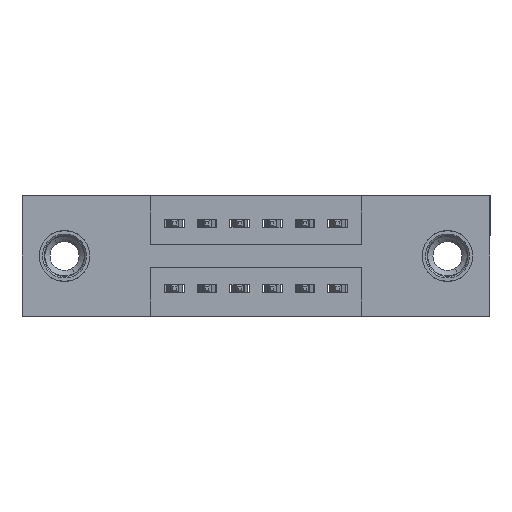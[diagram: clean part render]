
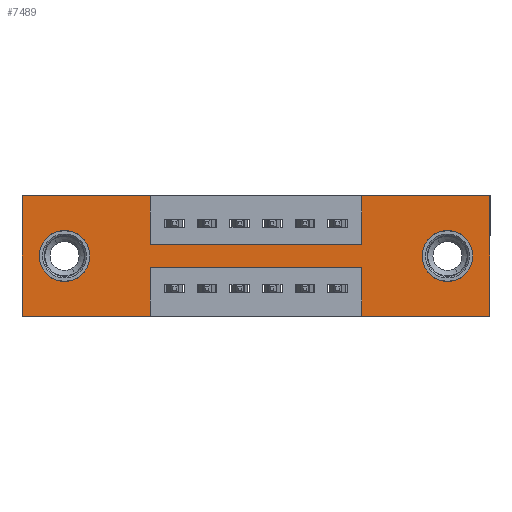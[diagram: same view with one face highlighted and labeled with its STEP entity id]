
A CAD part, front view. The second image highlights one B-rep face of the part: STEP entity #7489.
In plain terms, the highlighted planar face has unit normal (0, -1, 0).
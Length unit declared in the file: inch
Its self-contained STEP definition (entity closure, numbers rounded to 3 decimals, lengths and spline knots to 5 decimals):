
#26 = EDGE_CURVE ( 'NONE', #7139, #14259, #8707, .T. ) ;
#125 = ORIENTED_EDGE ( 'NONE', *, *, #11807, .F. ) ;
#130 = EDGE_CURVE ( 'NONE', #8347, #7900, #1981, .T. ) ;
#423 = VERTEX_POINT ( 'NONE', #5772 ) ;
#432 = LINE ( 'NONE', #14017, #3225 ) ;
#647 = DIRECTION ( 'NONE',  ( 0., 0., 1. ) ) ;
#673 = DIRECTION ( 'NONE',  ( 0., 0., 1. ) ) ;
#773 = VERTEX_POINT ( 'NONE', #10012 ) ;
#780 = DIRECTION ( 'NONE',  ( 1., 0., 0. ) ) ;
#805 = DIRECTION ( 'NONE',  ( 0., 0., -1. ) ) ;
#815 = VECTOR ( 'NONE', #3861, 39.37008 ) ;
#1123 = CARTESIAN_POINT ( 'NONE',  ( 0.3925, 0., -0.37 ) ) ;
#1194 = CARTESIAN_POINT ( 'NONE',  ( 0.3925, 0., 0. ) ) ;
#1325 = EDGE_CURVE ( 'NONE', #8647, #3098, #4925, .T. ) ;
#1399 = ORIENTED_EDGE ( 'NONE', *, *, #7856, .F. ) ;
#1472 = DIRECTION ( 'NONE',  ( -1., 0., 0. ) ) ;
#1557 = LINE ( 'NONE', #3007, #12269 ) ;
#1626 = AXIS2_PLACEMENT_3D ( 'NONE', #12969, #5193, #4157 ) ;
#1705 = ORIENTED_EDGE ( 'NONE', *, *, #10579, .F. ) ;
#1867 = CIRCLE ( 'NONE', #9782, 0.078 ) ;
#1916 = DIRECTION ( 'NONE',  ( 0., 0., -1. ) ) ;
#1981 = CIRCLE ( 'NONE', #10982, 0.078 ) ;
#1982 = VERTEX_POINT ( 'NONE', #1123 ) ;
#2013 = CARTESIAN_POINT ( 'NONE',  ( 1.0425, 0., 0. ) ) ;
#2030 = VECTOR ( 'NONE', #7546, 39.37008 ) ;
#2042 = DIRECTION ( 'NONE',  ( 0., 0., -1. ) ) ;
#2120 = CARTESIAN_POINT ( 'NONE',  ( 1.0425, 0., -0.22 ) ) ;
#2320 = CARTESIAN_POINT ( 'NONE',  ( 0., 0., 0. ) ) ;
#2398 = ORIENTED_EDGE ( 'NONE', *, *, #130, .T. ) ;
#2782 = CARTESIAN_POINT ( 'NONE',  ( 0.3925, 0., -0.22 ) ) ;
#2794 = CARTESIAN_POINT ( 'NONE',  ( 1.0425, 0., 0. ) ) ;
#2824 = EDGE_CURVE ( 'NONE', #14259, #8647, #2837, .T. ) ;
#2837 = LINE ( 'NONE', #7386, #13519 ) ;
#2948 = LINE ( 'NONE', #7271, #6345 ) ;
#3007 = CARTESIAN_POINT ( 'NONE',  ( 1.435, 0., 0. ) ) ;
#3098 = VERTEX_POINT ( 'NONE', #8872 ) ;
#3194 = CARTESIAN_POINT ( 'NONE',  ( 0.13, 0., -0.185 ) ) ;
#3225 = VECTOR ( 'NONE', #11664, 39.37008 ) ;
#3326 = DIRECTION ( 'NONE',  ( 0., 1., 0. ) ) ;
#3330 = ORIENTED_EDGE ( 'NONE', *, *, #9464, .T. ) ;
#3466 = CARTESIAN_POINT ( 'NONE',  ( 1.305, 0., -0.263 ) ) ;
#3505 = CARTESIAN_POINT ( 'NONE',  ( 1.305, 0., -0.185 ) ) ;
#3598 = CARTESIAN_POINT ( 'NONE',  ( 1.0425, 0., -0.37 ) ) ;
#3642 = DIRECTION ( 'NONE',  ( 0., 1., 0. ) ) ;
#3861 = DIRECTION ( 'NONE',  ( -1., 0., 0. ) ) ;
#4094 = FACE_OUTER_BOUND ( 'NONE', #10995, .T. ) ;
#4157 = DIRECTION ( 'NONE',  ( 0., 0., -1. ) ) ;
#4334 = AXIS2_PLACEMENT_3D ( 'NONE', #3505, #3642, #7861 ) ;
#4424 = LINE ( 'NONE', #9378, #815 ) ;
#4527 = VECTOR ( 'NONE', #2042, 39.37008 ) ;
#4878 = VERTEX_POINT ( 'NONE', #7983 ) ;
#4925 = LINE ( 'NONE', #9802, #2030 ) ;
#4985 = ORIENTED_EDGE ( 'NONE', *, *, #6591, .F. ) ;
#5040 = CIRCLE ( 'NONE', #6045, 0.078 ) ;
#5052 = CARTESIAN_POINT ( 'NONE',  ( 0.13, 0., -0.107 ) ) ;
#5193 = DIRECTION ( 'NONE',  ( 0., -1., 0. ) ) ;
#5353 = ORIENTED_EDGE ( 'NONE', *, *, #13831, .F. ) ;
#5372 = ORIENTED_EDGE ( 'NONE', *, *, #7749, .F. ) ;
#5481 = VECTOR ( 'NONE', #9433, 39.37008 ) ;
#5742 = LINE ( 'NONE', #10903, #4527 ) ;
#5757 = EDGE_CURVE ( 'NONE', #7882, #13334, #2948, .T. ) ;
#5772 = CARTESIAN_POINT ( 'NONE',  ( 0.3925, 0., -0.22 ) ) ;
#6045 = AXIS2_PLACEMENT_3D ( 'NONE', #6764, #3326, #6701 ) ;
#6271 = CARTESIAN_POINT ( 'NONE',  ( 1.305, 0., -0.107 ) ) ;
#6345 = VECTOR ( 'NONE', #673, 39.37008 ) ;
#6355 = DIRECTION ( 'NONE',  ( 0., 1., 0. ) ) ;
#6416 = ORIENTED_EDGE ( 'NONE', *, *, #26, .F. ) ;
#6497 = CIRCLE ( 'NONE', #4334, 0.078 ) ;
#6591 = EDGE_CURVE ( 'NONE', #3098, #11166, #8926, .T. ) ;
#6701 = DIRECTION ( 'NONE',  ( 0., 0., 1. ) ) ;
#6764 = CARTESIAN_POINT ( 'NONE',  ( 0.13, 0., -0.185 ) ) ;
#6765 = VERTEX_POINT ( 'NONE', #2013 ) ;
#7080 = VERTEX_POINT ( 'NONE', #5052 ) ;
#7139 = VERTEX_POINT ( 'NONE', #8402 ) ;
#7271 = CARTESIAN_POINT ( 'NONE',  ( 1.0425, 0., -0.37 ) ) ;
#7325 = VECTOR ( 'NONE', #647, 39.37008 ) ;
#7386 = CARTESIAN_POINT ( 'NONE',  ( 0., 0., 0. ) ) ;
#7418 = EDGE_CURVE ( 'NONE', #10824, #7080, #1867, .T. ) ;
#7489 = ADVANCED_FACE ( 'NONE', ( #8905, #12936, #4094 ), #8713, .T. ) ;
#7546 = DIRECTION ( 'NONE',  ( 0., 0., -1. ) ) ;
#7749 = EDGE_CURVE ( 'NONE', #6765, #773, #432, .T. ) ;
#7801 = ORIENTED_EDGE ( 'NONE', *, *, #9927, .F. ) ;
#7856 = EDGE_CURVE ( 'NONE', #4878, #7882, #8891, .T. ) ;
#7861 = DIRECTION ( 'NONE',  ( 0., 0., -1. ) ) ;
#7882 = VERTEX_POINT ( 'NONE', #3598 ) ;
#7900 = VERTEX_POINT ( 'NONE', #3466 ) ;
#7983 = CARTESIAN_POINT ( 'NONE',  ( 1.435, 0., -0.37 ) ) ;
#8144 = ORIENTED_EDGE ( 'NONE', *, *, #12425, .F. ) ;
#8347 = VERTEX_POINT ( 'NONE', #6271 ) ;
#8402 = CARTESIAN_POINT ( 'NONE',  ( 0., 0., -0.37 ) ) ;
#8422 = VECTOR ( 'NONE', #12541, 39.37008 ) ;
#8647 = VERTEX_POINT ( 'NONE', #1194 ) ;
#8707 = LINE ( 'NONE', #13751, #7325 ) ;
#8713 = PLANE ( 'NONE',  #1626 ) ;
#8872 = CARTESIAN_POINT ( 'NONE',  ( 0.3925, 0., -0.15 ) ) ;
#8891 = LINE ( 'NONE', #10269, #10285 ) ;
#8905 = FACE_BOUND ( 'NONE', #13918, .T. ) ;
#8926 = LINE ( 'NONE', #10300, #8422 ) ;
#8927 = VECTOR ( 'NONE', #10356, 39.37008 ) ;
#9076 = CARTESIAN_POINT ( 'NONE',  ( 1.0425, 0., -0.15 ) ) ;
#9378 = CARTESIAN_POINT ( 'NONE',  ( 0., 0., -0.37 ) ) ;
#9433 = DIRECTION ( 'NONE',  ( -1., 0., 0. ) ) ;
#9464 = EDGE_CURVE ( 'NONE', #7080, #10824, #5040, .T. ) ;
#9762 = DIRECTION ( 'NONE',  ( 0., 0., 1. ) ) ;
#9782 = AXIS2_PLACEMENT_3D ( 'NONE', #3194, #9800, #9762 ) ;
#9800 = DIRECTION ( 'NONE',  ( 0., 1., 0. ) ) ;
#9802 = CARTESIAN_POINT ( 'NONE',  ( 0.3925, 0., 0. ) ) ;
#9927 = EDGE_CURVE ( 'NONE', #423, #1982, #5742, .T. ) ;
#10012 = CARTESIAN_POINT ( 'NONE',  ( 1.435, 0., 0. ) ) ;
#10254 = CARTESIAN_POINT ( 'NONE',  ( 0.13, 0., -0.263 ) ) ;
#10269 = CARTESIAN_POINT ( 'NONE',  ( 0., 0., -0.37 ) ) ;
#10285 = VECTOR ( 'NONE', #1472, 39.37008 ) ;
#10300 = CARTESIAN_POINT ( 'NONE',  ( 0.3925, 0., -0.15 ) ) ;
#10356 = DIRECTION ( 'NONE',  ( 0., 0., 1. ) ) ;
#10579 = EDGE_CURVE ( 'NONE', #773, #4878, #1557, .T. ) ;
#10824 = VERTEX_POINT ( 'NONE', #10254 ) ;
#10903 = CARTESIAN_POINT ( 'NONE',  ( 0.3925, 0., -0.37 ) ) ;
#10982 = AXIS2_PLACEMENT_3D ( 'NONE', #14202, #6355, #1916 ) ;
#10995 = EDGE_LOOP ( 'NONE', ( #7801, #5353, #13824, #1399, #1705, #5372, #125, #4985, #11221, #11228, #6416, #8144 ) ) ;
#11050 = LINE ( 'NONE', #2782, #5481 ) ;
#11166 = VERTEX_POINT ( 'NONE', #9076 ) ;
#11221 = ORIENTED_EDGE ( 'NONE', *, *, #1325, .F. ) ;
#11228 = ORIENTED_EDGE ( 'NONE', *, *, #2824, .F. ) ;
#11500 = EDGE_LOOP ( 'NONE', ( #3330, #11600 ) ) ;
#11600 = ORIENTED_EDGE ( 'NONE', *, *, #7418, .T. ) ;
#11664 = DIRECTION ( 'NONE',  ( 1., 0., 0. ) ) ;
#11807 = EDGE_CURVE ( 'NONE', #11166, #6765, #13630, .T. ) ;
#12183 = EDGE_CURVE ( 'NONE', #7900, #8347, #6497, .T. ) ;
#12269 = VECTOR ( 'NONE', #805, 39.37008 ) ;
#12425 = EDGE_CURVE ( 'NONE', #1982, #7139, #4424, .T. ) ;
#12541 = DIRECTION ( 'NONE',  ( 1., 0., 0. ) ) ;
#12936 = FACE_BOUND ( 'NONE', #11500, .T. ) ;
#12969 = CARTESIAN_POINT ( 'NONE',  ( 0., 0., -0.37 ) ) ;
#13334 = VERTEX_POINT ( 'NONE', #2120 ) ;
#13338 = ORIENTED_EDGE ( 'NONE', *, *, #12183, .T. ) ;
#13519 = VECTOR ( 'NONE', #780, 39.37008 ) ;
#13630 = LINE ( 'NONE', #2794, #8927 ) ;
#13751 = CARTESIAN_POINT ( 'NONE',  ( 0., 0., 0. ) ) ;
#13824 = ORIENTED_EDGE ( 'NONE', *, *, #5757, .F. ) ;
#13831 = EDGE_CURVE ( 'NONE', #13334, #423, #11050, .T. ) ;
#13918 = EDGE_LOOP ( 'NONE', ( #2398, #13338 ) ) ;
#14017 = CARTESIAN_POINT ( 'NONE',  ( 0., 0., 0. ) ) ;
#14202 = CARTESIAN_POINT ( 'NONE',  ( 1.305, 0., -0.185 ) ) ;
#14259 = VERTEX_POINT ( 'NONE', #2320 ) ;
